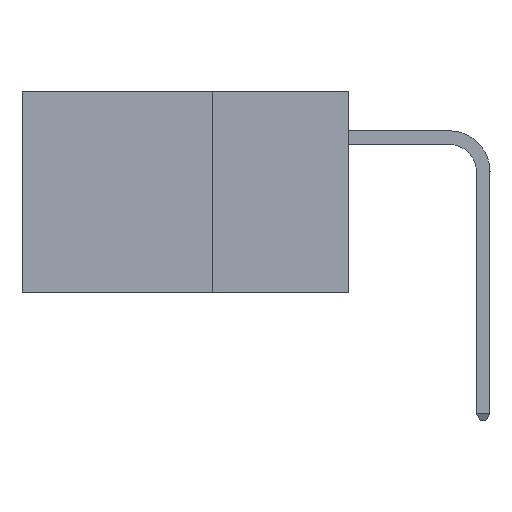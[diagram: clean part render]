
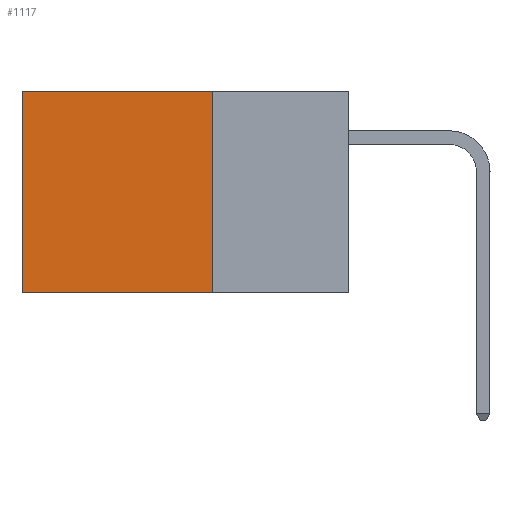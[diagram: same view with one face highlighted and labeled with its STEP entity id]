
A CAD part, left-side view. The second image highlights one B-rep face of the part: STEP entity #1117.
In plain terms, the highlighted planar face has unit normal (-1, 0, 0).
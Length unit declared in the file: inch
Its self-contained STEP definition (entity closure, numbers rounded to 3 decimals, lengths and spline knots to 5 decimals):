
#658 = CARTESIAN_POINT ( 'NONE',  ( 0.2875, 0.25, -0.37 ) ) ;
#722 = EDGE_CURVE ( 'NONE', #4460, #7454, #5194, .T. ) ;
#1019 = DIRECTION ( 'NONE',  ( 0., 0., -1. ) ) ;
#1117 = ADVANCED_FACE ( 'NONE', ( #3402 ), #7686, .F. ) ;
#1447 = AXIS2_PLACEMENT_3D ( 'NONE', #7580, #7511, #7491 ) ;
#1575 = VERTEX_POINT ( 'NONE', #658 ) ;
#2150 = VECTOR ( 'NONE', #10496, 39.37008 ) ;
#2320 = VECTOR ( 'NONE', #2475, 39.37008 ) ;
#2363 = LINE ( 'NONE', #2441, #2320 ) ;
#2441 = CARTESIAN_POINT ( 'NONE',  ( 0.2875, 0.25, 0. ) ) ;
#2475 = DIRECTION ( 'NONE',  ( 0., 1., 0. ) ) ;
#3402 = FACE_OUTER_BOUND ( 'NONE', #10589, .T. ) ;
#3780 = EDGE_CURVE ( 'NONE', #10495, #4460, #2363, .T. ) ;
#3904 = CARTESIAN_POINT ( 'NONE',  ( 0.2875, 0.6, -0.37 ) ) ;
#4460 = VERTEX_POINT ( 'NONE', #10929 ) ;
#4630 = DIRECTION ( 'NONE',  ( 0., 1., 0. ) ) ;
#5194 = LINE ( 'NONE', #10596, #5478 ) ;
#5235 = LINE ( 'NONE', #5898, #2150 ) ;
#5478 = VECTOR ( 'NONE', #1019, 39.37008 ) ;
#5898 = CARTESIAN_POINT ( 'NONE',  ( 0.2875, 0.25, 0. ) ) ;
#7081 = LINE ( 'NONE', #8821, #10755 ) ;
#7454 = VERTEX_POINT ( 'NONE', #3904 ) ;
#7491 = DIRECTION ( 'NONE',  ( 0., 0., -1. ) ) ;
#7511 = DIRECTION ( 'NONE',  ( 1., 0., 0. ) ) ;
#7580 = CARTESIAN_POINT ( 'NONE',  ( 0.2875, 0.25, 0. ) ) ;
#7686 = PLANE ( 'NONE',  #1447 ) ;
#8096 = ORIENTED_EDGE ( 'NONE', *, *, #722, .T. ) ;
#8392 = EDGE_CURVE ( 'NONE', #1575, #7454, #7081, .T. ) ;
#8584 = ORIENTED_EDGE ( 'NONE', *, *, #3780, .T. ) ;
#8821 = CARTESIAN_POINT ( 'NONE',  ( 0.2875, 0.25, -0.37 ) ) ;
#9380 = CARTESIAN_POINT ( 'NONE',  ( 0.2875, 0.25, 0. ) ) ;
#10170 = ORIENTED_EDGE ( 'NONE', *, *, #8392, .F. ) ;
#10238 = ORIENTED_EDGE ( 'NONE', *, *, #10855, .F. ) ;
#10495 = VERTEX_POINT ( 'NONE', #9380 ) ;
#10496 = DIRECTION ( 'NONE',  ( 0., 0., -1. ) ) ;
#10589 = EDGE_LOOP ( 'NONE', ( #8096, #10170, #10238, #8584 ) ) ;
#10596 = CARTESIAN_POINT ( 'NONE',  ( 0.2875, 0.6, 0. ) ) ;
#10755 = VECTOR ( 'NONE', #4630, 39.37008 ) ;
#10855 = EDGE_CURVE ( 'NONE', #10495, #1575, #5235, .T. ) ;
#10929 = CARTESIAN_POINT ( 'NONE',  ( 0.2875, 0.6, 0. ) ) ;
